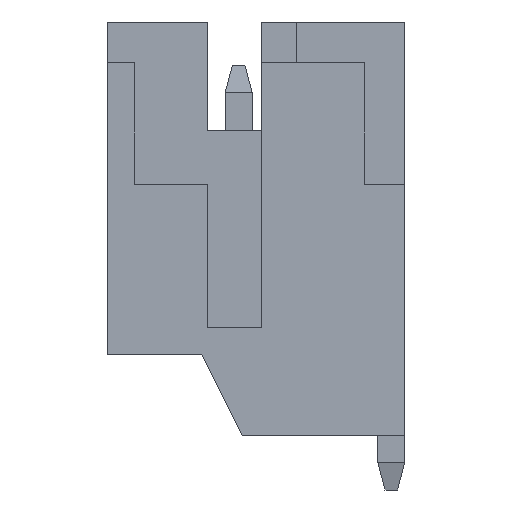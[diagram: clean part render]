
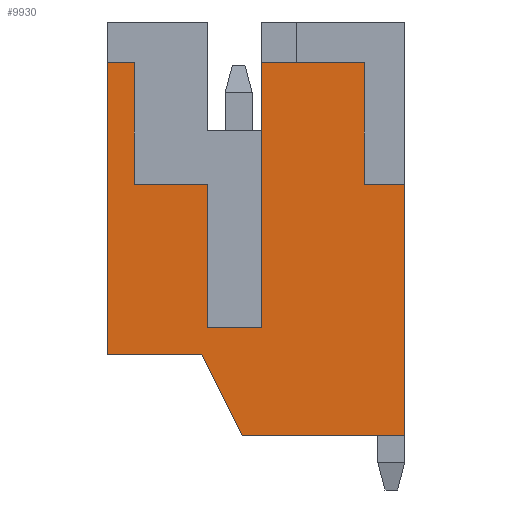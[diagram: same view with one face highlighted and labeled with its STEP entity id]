
A CAD part, left-side view. The second image highlights one B-rep face of the part: STEP entity #9930.
In plain terms, the highlighted planar face has unit normal (-1, 0, 0).
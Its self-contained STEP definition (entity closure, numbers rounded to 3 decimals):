
#132 = CARTESIAN_POINT ( 'NONE',  ( -3., 0.68, 0. ) ) ;
#172 = VECTOR ( 'NONE', #3748, 1000. ) ;
#826 = VERTEX_POINT ( 'NONE', #1052 ) ;
#882 = ORIENTED_EDGE ( 'NONE', *, *, #8487, .T. ) ;
#1052 = CARTESIAN_POINT ( 'NONE',  ( -3., 1.93, 5.4 ) ) ;
#1332 = VERTEX_POINT ( 'NONE', #7486 ) ;
#1484 = CARTESIAN_POINT ( 'NONE',  ( -3., -2.32, 3.15 ) ) ;
#1555 = CARTESIAN_POINT ( 'NONE',  ( -3., 1.93, 3.15 ) ) ;
#1913 = CARTESIAN_POINT ( 'NONE',  ( -3., -0.42, 6.15 ) ) ;
#1928 = ORIENTED_EDGE ( 'NONE', *, *, #7847, .F. ) ;
#1956 = LINE ( 'NONE', #5116, #3883 ) ;
#2251 = CARTESIAN_POINT ( 'NONE',  ( -3., -3.07, 5.4 ) ) ;
#2360 = LINE ( 'NONE', #2631, #6771 ) ;
#2631 = CARTESIAN_POINT ( 'NONE',  ( -3., -3.07, -1.5 ) ) ;
#2634 = CARTESIAN_POINT ( 'NONE',  ( -3., -2.32, 3.15 ) ) ;
#2653 = DIRECTION ( 'NONE',  ( 0., -0.447, -0.894 ) ) ;
#2687 = DIRECTION ( 'NONE',  ( 0., 0., -1. ) ) ;
#2726 = EDGE_CURVE ( 'NONE', #826, #5485, #1956, .T. ) ;
#2745 = VECTOR ( 'NONE', #2653, 1000. ) ;
#2868 = CARTESIAN_POINT ( 'NONE',  ( -3., -3.07, 6.15 ) ) ;
#2896 = LINE ( 'NONE', #8016, #2745 ) ;
#2918 = LINE ( 'NONE', #2634, #6358 ) ;
#2920 = CARTESIAN_POINT ( 'NONE',  ( -3., -0.42, 0.5 ) ) ;
#2949 = EDGE_CURVE ( 'NONE', #8710, #4865, #2918, .T. ) ;
#3007 = DIRECTION ( 'NONE',  ( 0., -1., 0. ) ) ;
#3020 = DIRECTION ( 'NONE',  ( 0., 0., -1. ) ) ;
#3033 = DIRECTION ( 'NONE',  ( 0., -1., 0. ) ) ;
#3053 = VERTEX_POINT ( 'NONE', #132 ) ;
#3174 = ORIENTED_EDGE ( 'NONE', *, *, #9712, .T. ) ;
#3190 = VERTEX_POINT ( 'NONE', #4050 ) ;
#3197 = CARTESIAN_POINT ( 'NONE',  ( -3., -2.32, 3.15 ) ) ;
#3401 = CARTESIAN_POINT ( 'NONE',  ( -3., 1.93, 3.15 ) ) ;
#3430 = LINE ( 'NONE', #5609, #7289 ) ;
#3447 = CARTESIAN_POINT ( 'NONE',  ( -3., 0.58, 0.5 ) ) ;
#3563 = ORIENTED_EDGE ( 'NONE', *, *, #4371, .F. ) ;
#3745 = CARTESIAN_POINT ( 'NONE',  ( -3., -0.42, 0.5 ) ) ;
#3748 = DIRECTION ( 'NONE',  ( 0., 0., 1. ) ) ;
#3765 = LINE ( 'NONE', #2868, #172 ) ;
#3826 = EDGE_CURVE ( 'NONE', #3053, #8222, #2896, .T. ) ;
#3847 = EDGE_CURVE ( 'NONE', #6384, #10966, #11472, .T. ) ;
#3883 = VECTOR ( 'NONE', #9620, 1000. ) ;
#3891 = VECTOR ( 'NONE', #11203, 1000. ) ;
#3996 = DIRECTION ( 'NONE',  ( -1., 0., 0. ) ) ;
#4050 = CARTESIAN_POINT ( 'NONE',  ( -3., 2.43, 0. ) ) ;
#4154 = VECTOR ( 'NONE', #7433, 1000. ) ;
#4240 = DIRECTION ( 'NONE',  ( 0., 0., 1. ) ) ;
#4371 = EDGE_CURVE ( 'NONE', #6336, #10966, #5761, .T. ) ;
#4454 = VECTOR ( 'NONE', #4240, 1000. ) ;
#4498 = EDGE_CURVE ( 'NONE', #10710, #6721, #3430, .T. ) ;
#4546 = CARTESIAN_POINT ( 'NONE',  ( -3., 2.43, 6.15 ) ) ;
#4640 = DIRECTION ( 'NONE',  ( 0., -1., 0. ) ) ;
#4737 = EDGE_LOOP ( 'NONE', ( #7602, #5338, #3174, #11288, #882, #6823, #10233, #5883, #11284, #9211, #3563, #1928, #11092, #4740 ) ) ;
#4740 = ORIENTED_EDGE ( 'NONE', *, *, #6952, .T. ) ;
#4865 = VERTEX_POINT ( 'NONE', #10740 ) ;
#4915 = PLANE ( 'NONE',  #6573 ) ;
#4920 = VECTOR ( 'NONE', #4640, 1000. ) ;
#5116 = CARTESIAN_POINT ( 'NONE',  ( -3., -3.07, 5.4 ) ) ;
#5261 = LINE ( 'NONE', #3197, #3891 ) ;
#5338 = ORIENTED_EDGE ( 'NONE', *, *, #9107, .T. ) ;
#5485 = VERTEX_POINT ( 'NONE', #11077 ) ;
#5609 = CARTESIAN_POINT ( 'NONE',  ( -3., -0.42, 3.15 ) ) ;
#5761 = LINE ( 'NONE', #2920, #4920 ) ;
#5883 = ORIENTED_EDGE ( 'NONE', *, *, #7609, .T. ) ;
#5902 = VECTOR ( 'NONE', #7331, 1000. ) ;
#6060 = CARTESIAN_POINT ( 'NONE',  ( -3., -0.42, 5.4 ) ) ;
#6324 = CARTESIAN_POINT ( 'NONE',  ( -3., -2.32, 5.4 ) ) ;
#6336 = VERTEX_POINT ( 'NONE', #3447 ) ;
#6358 = VECTOR ( 'NONE', #10633, 1000. ) ;
#6384 = VERTEX_POINT ( 'NONE', #6060 ) ;
#6541 = LINE ( 'NONE', #3401, #4454 ) ;
#6573 = AXIS2_PLACEMENT_3D ( 'NONE', #10101, #3996, #3007 ) ;
#6583 = EDGE_CURVE ( 'NONE', #1332, #4865, #3765, .T. ) ;
#6721 = VERTEX_POINT ( 'NONE', #8262 ) ;
#6771 = VECTOR ( 'NONE', #10747, 1000. ) ;
#6823 = ORIENTED_EDGE ( 'NONE', *, *, #6583, .T. ) ;
#6843 = CARTESIAN_POINT ( 'NONE',  ( -3., -0.07, -1.5 ) ) ;
#6952 = EDGE_CURVE ( 'NONE', #10710, #826, #6541, .T. ) ;
#7289 = VECTOR ( 'NONE', #3033, 1000. ) ;
#7331 = DIRECTION ( 'NONE',  ( 0., -1., 0. ) ) ;
#7433 = DIRECTION ( 'NONE',  ( 0., 1., 0. ) ) ;
#7486 = CARTESIAN_POINT ( 'NONE',  ( -3., -3.07, -1.5 ) ) ;
#7586 = LINE ( 'NONE', #4546, #8822 ) ;
#7602 = ORIENTED_EDGE ( 'NONE', *, *, #2726, .T. ) ;
#7609 = EDGE_CURVE ( 'NONE', #8710, #8539, #5261, .T. ) ;
#7847 = EDGE_CURVE ( 'NONE', #6721, #6336, #8997, .T. ) ;
#8016 = CARTESIAN_POINT ( 'NONE',  ( -3., -0.07, -1.5 ) ) ;
#8198 = EDGE_CURVE ( 'NONE', #8539, #6384, #10387, .T. ) ;
#8222 = VERTEX_POINT ( 'NONE', #6843 ) ;
#8262 = CARTESIAN_POINT ( 'NONE',  ( -3., 0.58, 3.15 ) ) ;
#8487 = EDGE_CURVE ( 'NONE', #8222, #1332, #2360, .T. ) ;
#8539 = VERTEX_POINT ( 'NONE', #6324 ) ;
#8710 = VERTEX_POINT ( 'NONE', #1484 ) ;
#8817 = CARTESIAN_POINT ( 'NONE',  ( -3., 0.58, 3.15 ) ) ;
#8822 = VECTOR ( 'NONE', #3020, 1000. ) ;
#8997 = LINE ( 'NONE', #8817, #11087 ) ;
#9098 = DIRECTION ( 'NONE',  ( 0., 0., -1. ) ) ;
#9107 = EDGE_CURVE ( 'NONE', #5485, #3190, #7586, .T. ) ;
#9211 = ORIENTED_EDGE ( 'NONE', *, *, #3847, .T. ) ;
#9620 = DIRECTION ( 'NONE',  ( 0., 1., 0. ) ) ;
#9712 = EDGE_CURVE ( 'NONE', #3190, #3053, #11185, .T. ) ;
#9789 = FACE_OUTER_BOUND ( 'NONE', #4737, .T. ) ;
#9930 = ADVANCED_FACE ( 'NONE', ( #9789 ), #4915, .T. ) ;
#10101 = CARTESIAN_POINT ( 'NONE',  ( -3., 0., 0. ) ) ;
#10233 = ORIENTED_EDGE ( 'NONE', *, *, #2949, .F. ) ;
#10387 = LINE ( 'NONE', #2251, #4154 ) ;
#10633 = DIRECTION ( 'NONE',  ( 0., -1., 0. ) ) ;
#10710 = VERTEX_POINT ( 'NONE', #1555 ) ;
#10740 = CARTESIAN_POINT ( 'NONE',  ( -3., -3.07, 3.15 ) ) ;
#10747 = DIRECTION ( 'NONE',  ( 0., -1., 0. ) ) ;
#10768 = CARTESIAN_POINT ( 'NONE',  ( -3., 2.43, 0. ) ) ;
#10921 = VECTOR ( 'NONE', #9098, 1000. ) ;
#10966 = VERTEX_POINT ( 'NONE', #3745 ) ;
#11077 = CARTESIAN_POINT ( 'NONE',  ( -3., 2.43, 5.4 ) ) ;
#11087 = VECTOR ( 'NONE', #2687, 1000. ) ;
#11092 = ORIENTED_EDGE ( 'NONE', *, *, #4498, .F. ) ;
#11185 = LINE ( 'NONE', #10768, #5902 ) ;
#11203 = DIRECTION ( 'NONE',  ( 0., 0., 1. ) ) ;
#11284 = ORIENTED_EDGE ( 'NONE', *, *, #8198, .T. ) ;
#11288 = ORIENTED_EDGE ( 'NONE', *, *, #3826, .T. ) ;
#11472 = LINE ( 'NONE', #1913, #10921 ) ;
